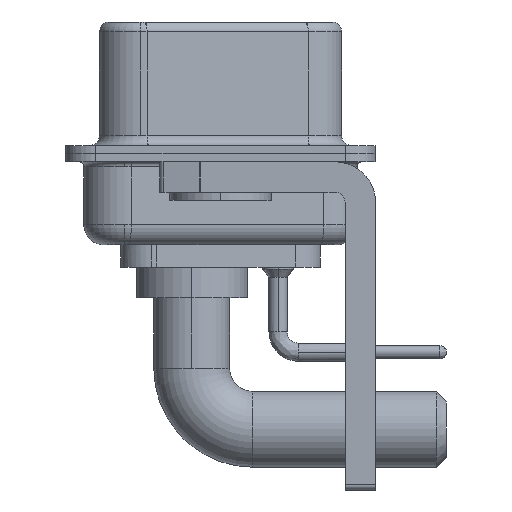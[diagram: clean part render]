
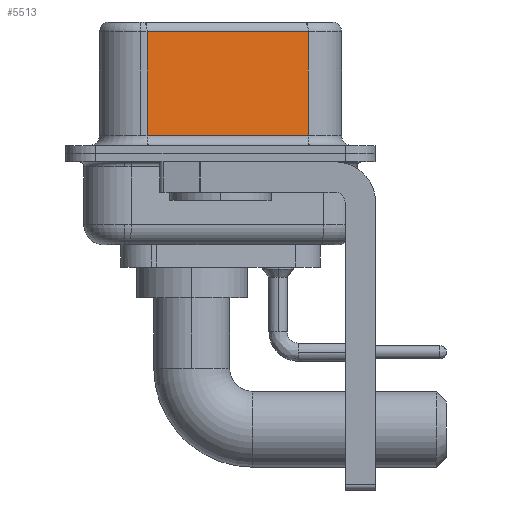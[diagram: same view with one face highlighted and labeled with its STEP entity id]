
A CAD part, left-side view. The second image highlights one B-rep face of the part: STEP entity #5513.
In plain terms, the highlighted planar face has unit normal (-0.985, -0.174, 0).
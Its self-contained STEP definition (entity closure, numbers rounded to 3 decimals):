
#784 = DIRECTION ( 'NONE',  ( -0.174, 0.985, 0. ) ) ;
#1161 = VECTOR ( 'NONE', #784, 1000. ) ;
#3024 = CARTESIAN_POINT ( 'NONE',  ( 5.132, -4.322, 6.02 ) ) ;
#3230 = EDGE_LOOP ( 'NONE', ( #9090, #11649, #21077, #17236 ) ) ;
#4912 = EDGE_CURVE ( 'NONE', #18322, #5633, #12801, .T. ) ;
#5513 = ADVANCED_FACE ( 'NONE', ( #19470 ), #17613, .F. ) ;
#5633 = VERTEX_POINT ( 'NONE', #6087 ) ;
#5641 = CARTESIAN_POINT ( 'NONE',  ( 3.73, 3.628, 6.02 ) ) ;
#6087 = CARTESIAN_POINT ( 'NONE',  ( 3.73, 3.628, 0.9 ) ) ;
#6291 = LINE ( 'NONE', #15752, #14653 ) ;
#6604 = LINE ( 'NONE', #20073, #7209 ) ;
#7209 = VECTOR ( 'NONE', #14211, 1000. ) ;
#7815 = DIRECTION ( 'NONE',  ( -0.174, 0.985, 0. ) ) ;
#8119 = CARTESIAN_POINT ( 'NONE',  ( 5.132, -4.322, 6.52 ) ) ;
#8129 = LINE ( 'NONE', #3024, #1161 ) ;
#8144 = EDGE_CURVE ( 'NONE', #8692, #18322, #8129, .T. ) ;
#8692 = VERTEX_POINT ( 'NONE', #12588 ) ;
#9090 = ORIENTED_EDGE ( 'NONE', *, *, #15744, .F. ) ;
#10154 = DIRECTION ( 'NONE',  ( 0.174, -0.985, 0. ) ) ;
#10824 = CARTESIAN_POINT ( 'NONE',  ( 3.73, 3.628, 6.52 ) ) ;
#11649 = ORIENTED_EDGE ( 'NONE', *, *, #8144, .T. ) ;
#12588 = CARTESIAN_POINT ( 'NONE',  ( 5.132, -4.322, 6.02 ) ) ;
#12801 = LINE ( 'NONE', #10824, #14181 ) ;
#14181 = VECTOR ( 'NONE', #22534, 1000. ) ;
#14199 = AXIS2_PLACEMENT_3D ( 'NONE', #8119, #15726, #7815 ) ;
#14211 = DIRECTION ( 'NONE',  ( 0., 0., -1. ) ) ;
#14653 = VECTOR ( 'NONE', #10154, 1000. ) ;
#15726 = DIRECTION ( 'NONE',  ( 0.985, 0.174, 0. ) ) ;
#15744 = EDGE_CURVE ( 'NONE', #8692, #23721, #6604, .T. ) ;
#15752 = CARTESIAN_POINT ( 'NONE',  ( 5.132, -4.322, 0.9 ) ) ;
#17236 = ORIENTED_EDGE ( 'NONE', *, *, #24016, .T. ) ;
#17613 = PLANE ( 'NONE',  #14199 ) ;
#17827 = CARTESIAN_POINT ( 'NONE',  ( 5.132, -4.322, 0.9 ) ) ;
#18322 = VERTEX_POINT ( 'NONE', #5641 ) ;
#19470 = FACE_OUTER_BOUND ( 'NONE', #3230, .T. ) ;
#20073 = CARTESIAN_POINT ( 'NONE',  ( 5.132, -4.322, 6.52 ) ) ;
#21077 = ORIENTED_EDGE ( 'NONE', *, *, #4912, .T. ) ;
#22534 = DIRECTION ( 'NONE',  ( 0., 0., -1. ) ) ;
#23721 = VERTEX_POINT ( 'NONE', #17827 ) ;
#24016 = EDGE_CURVE ( 'NONE', #5633, #23721, #6291, .T. ) ;
